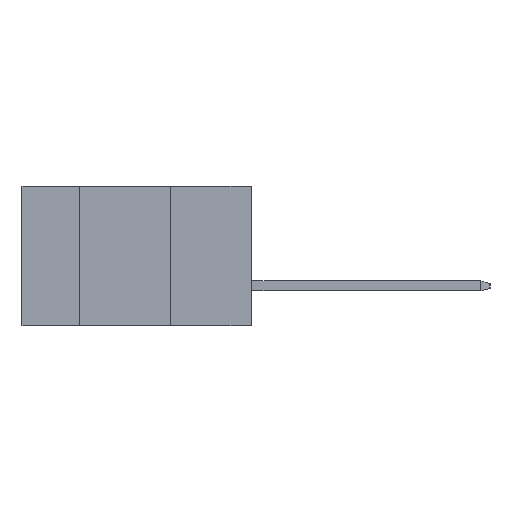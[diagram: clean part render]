
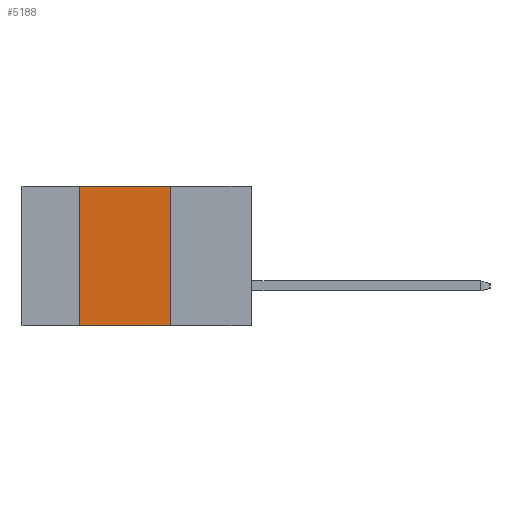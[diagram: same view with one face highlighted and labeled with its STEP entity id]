
A CAD part, left-side view. The second image highlights one B-rep face of the part: STEP entity #5188.
In plain terms, the highlighted planar face has unit normal (-1, 0, 0).
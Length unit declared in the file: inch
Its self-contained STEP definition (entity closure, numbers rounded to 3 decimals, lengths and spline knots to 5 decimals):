
#161 = CARTESIAN_POINT ( 'NONE',  ( 0., 0.254, -0.437 ) ) ;
#209 = FACE_OUTER_BOUND ( 'NONE', #3806, .T. ) ;
#342 = VECTOR ( 'NONE', #4500, 39.37008 ) ;
#657 = VECTOR ( 'NONE', #1440, 39.37008 ) ;
#806 = EDGE_CURVE ( 'NONE', #7602, #8261, #1728, .T. ) ;
#1391 = DIRECTION ( 'NONE',  ( 0., 0., 1. ) ) ;
#1440 = DIRECTION ( 'NONE',  ( 0., -1., 0. ) ) ;
#1484 = VERTEX_POINT ( 'NONE', #7570 ) ;
#1728 = LINE ( 'NONE', #3694, #342 ) ;
#2015 = EDGE_CURVE ( 'NONE', #8261, #5195, #3714, .T. ) ;
#2301 = DIRECTION ( 'NONE',  ( 0., 0., -1. ) ) ;
#2340 = DIRECTION ( 'NONE',  ( 0., 0., -1. ) ) ;
#2764 = CARTESIAN_POINT ( 'NONE',  ( 0., 0.54, -0.437 ) ) ;
#3276 = AXIS2_PLACEMENT_3D ( 'NONE', #7934, #4521, #2301 ) ;
#3577 = LINE ( 'NONE', #4351, #657 ) ;
#3694 = CARTESIAN_POINT ( 'NONE',  ( 0., 0.72, 0. ) ) ;
#3714 = LINE ( 'NONE', #161, #8429 ) ;
#3806 = EDGE_LOOP ( 'NONE', ( #3945, #5205, #7355, #6104 ) ) ;
#3945 = ORIENTED_EDGE ( 'NONE', *, *, #2015, .F. ) ;
#4351 = CARTESIAN_POINT ( 'NONE',  ( 0., 0.72, -0.437 ) ) ;
#4500 = DIRECTION ( 'NONE',  ( 0., -1., 0. ) ) ;
#4521 = DIRECTION ( 'NONE',  ( 1., 0., 0. ) ) ;
#4757 = VECTOR ( 'NONE', #1391, 39.37008 ) ;
#4990 = EDGE_CURVE ( 'NONE', #1484, #5195, #3577, .T. ) ;
#5188 = ADVANCED_FACE ( 'NONE', ( #209 ), #8619, .F. ) ;
#5195 = VERTEX_POINT ( 'NONE', #5209 ) ;
#5205 = ORIENTED_EDGE ( 'NONE', *, *, #806, .F. ) ;
#5209 = CARTESIAN_POINT ( 'NONE',  ( 0., 0.254, -0.437 ) ) ;
#6104 = ORIENTED_EDGE ( 'NONE', *, *, #4990, .T. ) ;
#7355 = ORIENTED_EDGE ( 'NONE', *, *, #7569, .F. ) ;
#7507 = CARTESIAN_POINT ( 'NONE',  ( 0., 0.254, 0. ) ) ;
#7569 = EDGE_CURVE ( 'NONE', #1484, #7602, #8985, .T. ) ;
#7570 = CARTESIAN_POINT ( 'NONE',  ( 0., 0.54, -0.437 ) ) ;
#7602 = VERTEX_POINT ( 'NONE', #8488 ) ;
#7934 = CARTESIAN_POINT ( 'NONE',  ( 0., 0.72, 0. ) ) ;
#8261 = VERTEX_POINT ( 'NONE', #7507 ) ;
#8429 = VECTOR ( 'NONE', #2340, 39.37008 ) ;
#8488 = CARTESIAN_POINT ( 'NONE',  ( 0., 0.54, 0. ) ) ;
#8619 = PLANE ( 'NONE',  #3276 ) ;
#8985 = LINE ( 'NONE', #2764, #4757 ) ;
